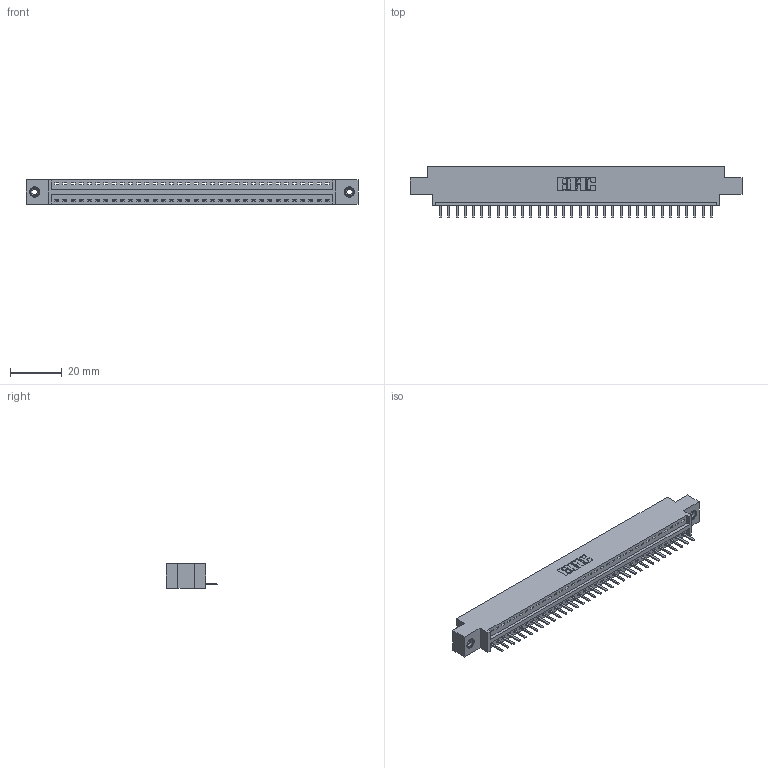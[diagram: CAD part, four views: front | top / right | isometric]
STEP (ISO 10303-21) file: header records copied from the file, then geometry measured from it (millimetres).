
FILE_DESCRIPTION (( 'STEP AP203' ), '1' );
FILE_NAME ('346-034-520-608.STEP', '2018-08-23T21:47:10', ( '' ), ( '' ), 'SwSTEP 2.0', 'SolidWorks 2016', '' );
FILE_SCHEMA (( 'CONFIG_CONTROL_DESIGN' ));
Length unit declared in the file: inch
Products named in the file (4): 345-250-001_345-250-003-102; 346-034-520-608; 346 Part_0.170 Offset - 0.156 Dia-TI; 345-292-001_345-293-120
Assembly tree (37 placements, depth 2):
  346-034-520-608
    346 Part_0.170 Offset - 0.156 Dia-TI
    345-292-001_345-293-120  x34
    345-250-001_345-250-003-102  x2
Bounding box: 128.52 x 20.02 x 9.4 mm (x, y, z)
Volume: 11988.5 mm3; surface area: 14753.5 mm2
Topology: 37 solids, 37 shells, 2294 faces, 6733 edges, 4390 vertices
Faces by surface type: plane 1540, cylinder 738, cone 12, torus 4
Entity records: 23610 total; most frequent: CARTESIAN_POINT 4045, ORIENTED_EDGE 3994, DIRECTION 3591, EDGE_CURVE 1997, LINE 1705, VECTOR 1705, VERTEX_POINT 1324, AXIS2_PLACEMENT_3D 943
